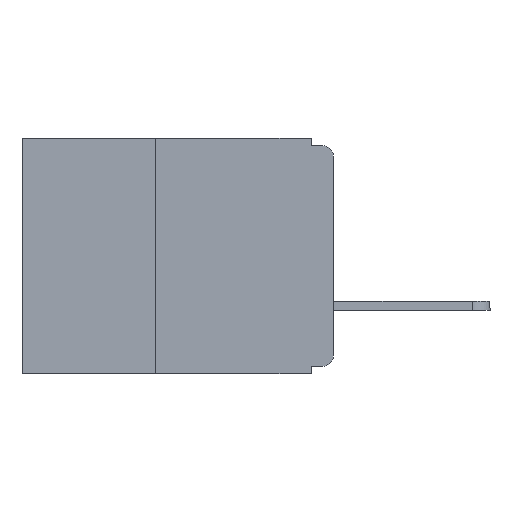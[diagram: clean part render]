
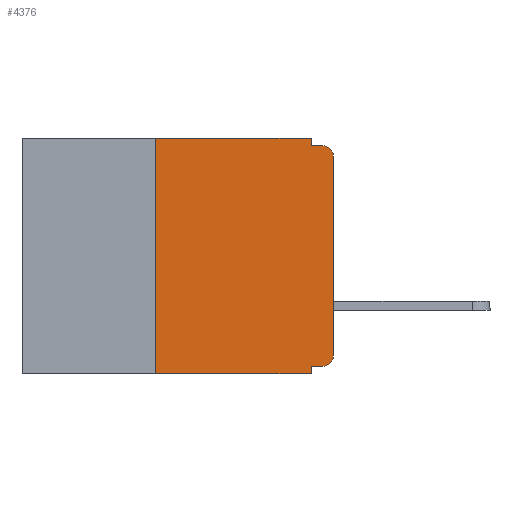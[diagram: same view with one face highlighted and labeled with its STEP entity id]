
A CAD part, left-side view. The second image highlights one B-rep face of the part: STEP entity #4376.
In plain terms, the highlighted planar face has unit normal (-1, 0, 0).
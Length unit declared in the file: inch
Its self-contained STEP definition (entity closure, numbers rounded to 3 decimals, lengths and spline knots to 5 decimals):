
#581 = VERTEX_POINT ( 'NONE', #13435 ) ;
#950 = VERTEX_POINT ( 'NONE', #9457 ) ;
#1292 = LINE ( 'NONE', #9750, #2821 ) ;
#1889 = EDGE_CURVE ( 'NONE', #14185, #12865, #10103, .T. ) ;
#2077 = VERTEX_POINT ( 'NONE', #4933 ) ;
#2437 = CARTESIAN_POINT ( 'NONE',  ( 0., 0.031, -0.01 ) ) ;
#2522 = CARTESIAN_POINT ( 'NONE',  ( 0., 0.015, -0.01 ) ) ;
#2821 = VECTOR ( 'NONE', #9371, 39.37008 ) ;
#3395 = VERTEX_POINT ( 'NONE', #10208 ) ;
#3508 = VECTOR ( 'NONE', #11872, 39.37008 ) ;
#3675 = LINE ( 'NONE', #16018, #3508 ) ;
#3863 = CARTESIAN_POINT ( 'NONE',  ( 0., 0., -0.305 ) ) ;
#4173 = VECTOR ( 'NONE', #15781, 39.37008 ) ;
#4197 = VECTOR ( 'NONE', #11992, 39.37008 ) ;
#4247 = LINE ( 'NONE', #12255, #4197 ) ;
#4376 = ADVANCED_FACE ( 'NONE', ( #10045 ), #16559, .F. ) ;
#4672 = LINE ( 'NONE', #10209, #4173 ) ;
#4730 = VECTOR ( 'NONE', #7651, 39.37008 ) ;
#4851 = LINE ( 'NONE', #8615, #4730 ) ;
#4933 = CARTESIAN_POINT ( 'NONE',  ( 0., 0., -0.025 ) ) ;
#5420 = VERTEX_POINT ( 'NONE', #3863 ) ;
#6090 = VECTOR ( 'NONE', #15532, 39.37008 ) ;
#6309 = EDGE_CURVE ( 'NONE', #5420, #2077, #9754, .T. ) ;
#7198 = EDGE_CURVE ( 'NONE', #581, #16651, #4247, .T. ) ;
#7410 = VECTOR ( 'NONE', #8587, 39.37008 ) ;
#7429 = EDGE_CURVE ( 'NONE', #12293, #12276, #1292, .T. ) ;
#7516 = LINE ( 'NONE', #15611, #6090 ) ;
#7651 = DIRECTION ( 'NONE',  ( 0., 0., -1. ) ) ;
#8016 = EDGE_CURVE ( 'NONE', #950, #581, #7516, .T. ) ;
#8205 = AXIS2_PLACEMENT_3D ( 'NONE', #15309, #14636, #14373 ) ;
#8390 = EDGE_CURVE ( 'NONE', #2077, #12276, #13647, .T. ) ;
#8443 = CARTESIAN_POINT ( 'NONE',  ( 0., 0., 0. ) ) ;
#8587 = DIRECTION ( 'NONE',  ( 0., 0., 1. ) ) ;
#8615 = CARTESIAN_POINT ( 'NONE',  ( 0., 0.031, 0. ) ) ;
#8739 = EDGE_CURVE ( 'NONE', #950, #5420, #17268, .T. ) ;
#9371 = DIRECTION ( 'NONE',  ( 0., -1., 0. ) ) ;
#9457 = CARTESIAN_POINT ( 'NONE',  ( 0., 0.015, -0.32 ) ) ;
#9549 = DIRECTION ( 'NONE',  ( 0., -1., 0. ) ) ;
#9715 = EDGE_LOOP ( 'NONE', ( #13242, #13258, #13446, #13641, #13725, #13813, #13897, #14233, #14276, #14527 ) ) ;
#9750 = CARTESIAN_POINT ( 'NONE',  ( 0., 0., -0.01 ) ) ;
#9754 = LINE ( 'NONE', #8443, #7410 ) ;
#10039 = VECTOR ( 'NONE', #9549, 39.37008 ) ;
#10045 = FACE_OUTER_BOUND ( 'NONE', #9715, .T. ) ;
#10103 = LINE ( 'NONE', #11032, #10039 ) ;
#10208 = CARTESIAN_POINT ( 'NONE',  ( 0., 0.25, -0.33 ) ) ;
#10209 = CARTESIAN_POINT ( 'NONE',  ( 0., 0.25, -0.33 ) ) ;
#11032 = CARTESIAN_POINT ( 'NONE',  ( 0., 0.437, 0. ) ) ;
#11872 = DIRECTION ( 'NONE',  ( 0., -1., 0. ) ) ;
#11945 = CARTESIAN_POINT ( 'NONE',  ( 0., 0.031, -0.33 ) ) ;
#11992 = DIRECTION ( 'NONE',  ( 0., 0., -1. ) ) ;
#12255 = CARTESIAN_POINT ( 'NONE',  ( 0., 0.031, -0.33 ) ) ;
#12276 = VERTEX_POINT ( 'NONE', #2522 ) ;
#12293 = VERTEX_POINT ( 'NONE', #2437 ) ;
#12865 = VERTEX_POINT ( 'NONE', #18051 ) ;
#13242 = ORIENTED_EDGE ( 'NONE', *, *, #6309, .T. ) ;
#13258 = ORIENTED_EDGE ( 'NONE', *, *, #8390, .T. ) ;
#13435 = CARTESIAN_POINT ( 'NONE',  ( 0., 0.031, -0.32 ) ) ;
#13446 = ORIENTED_EDGE ( 'NONE', *, *, #7429, .F. ) ;
#13641 = ORIENTED_EDGE ( 'NONE', *, *, #17672, .F. ) ;
#13647 = CIRCLE ( 'NONE', #8205, 0.015 ) ;
#13725 = ORIENTED_EDGE ( 'NONE', *, *, #1889, .F. ) ;
#13813 = ORIENTED_EDGE ( 'NONE', *, *, #17745, .F. ) ;
#13897 = ORIENTED_EDGE ( 'NONE', *, *, #17899, .T. ) ;
#14091 = AXIS2_PLACEMENT_3D ( 'NONE', #16616, #16179, #16134 ) ;
#14185 = VERTEX_POINT ( 'NONE', #14682 ) ;
#14233 = ORIENTED_EDGE ( 'NONE', *, *, #7198, .F. ) ;
#14276 = ORIENTED_EDGE ( 'NONE', *, *, #8016, .F. ) ;
#14373 = DIRECTION ( 'NONE',  ( 0., 0., -1. ) ) ;
#14527 = ORIENTED_EDGE ( 'NONE', *, *, #8739, .T. ) ;
#14636 = DIRECTION ( 'NONE',  ( -1., 0., 0. ) ) ;
#14682 = CARTESIAN_POINT ( 'NONE',  ( 0., 0.25, 0. ) ) ;
#15309 = CARTESIAN_POINT ( 'NONE',  ( 0., 0.015, -0.025 ) ) ;
#15532 = DIRECTION ( 'NONE',  ( 0., 1., 0. ) ) ;
#15611 = CARTESIAN_POINT ( 'NONE',  ( 0., 0., -0.32 ) ) ;
#15781 = DIRECTION ( 'NONE',  ( 0., 0., 1. ) ) ;
#15809 = DIRECTION ( 'NONE',  ( 0., 0., -1. ) ) ;
#15816 = DIRECTION ( 'NONE',  ( -1., 0., 0. ) ) ;
#15895 = CARTESIAN_POINT ( 'NONE',  ( 0., 0.015, -0.305 ) ) ;
#16018 = CARTESIAN_POINT ( 'NONE',  ( 0., 0.437, -0.33 ) ) ;
#16134 = DIRECTION ( 'NONE',  ( 0., 0., -1. ) ) ;
#16179 = DIRECTION ( 'NONE',  ( 1., 0., 0. ) ) ;
#16559 = PLANE ( 'NONE',  #14091 ) ;
#16616 = CARTESIAN_POINT ( 'NONE',  ( 0., 0.437, 0. ) ) ;
#16651 = VERTEX_POINT ( 'NONE', #11945 ) ;
#17268 = CIRCLE ( 'NONE', #18129, 0.015 ) ;
#17672 = EDGE_CURVE ( 'NONE', #12865, #12293, #4851, .T. ) ;
#17745 = EDGE_CURVE ( 'NONE', #3395, #14185, #4672, .T. ) ;
#17899 = EDGE_CURVE ( 'NONE', #3395, #16651, #3675, .T. ) ;
#18051 = CARTESIAN_POINT ( 'NONE',  ( 0., 0.031, 0. ) ) ;
#18129 = AXIS2_PLACEMENT_3D ( 'NONE', #15895, #15816, #15809 ) ;
